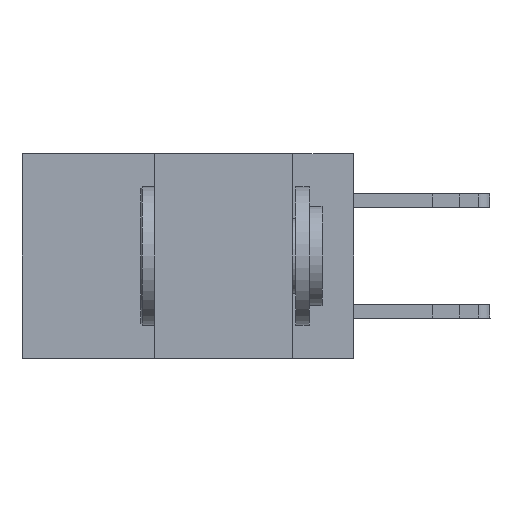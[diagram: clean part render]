
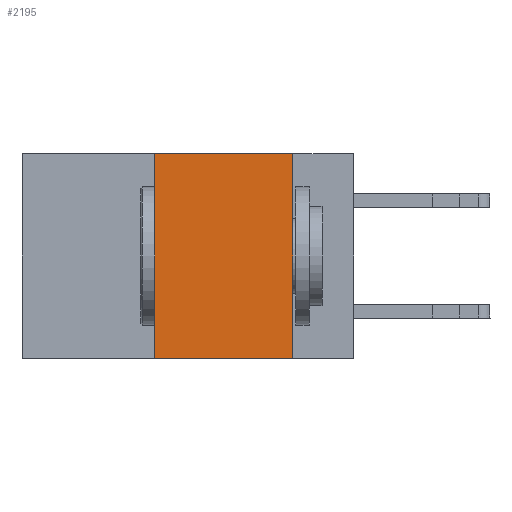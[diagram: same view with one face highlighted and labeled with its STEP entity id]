
A CAD part, left-side view. The second image highlights one B-rep face of the part: STEP entity #2195.
In plain terms, the highlighted planar face has unit normal (-1, 0, 0).
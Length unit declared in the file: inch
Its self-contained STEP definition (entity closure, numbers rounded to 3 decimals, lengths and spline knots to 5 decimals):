
#376 = DIRECTION ( 'NONE',  ( 0., 0., -1. ) ) ;
#899 = CARTESIAN_POINT ( 'NONE',  ( 0., 0.36, 0. ) ) ;
#1220 = VECTOR ( 'NONE', #376, 39.37008 ) ;
#1946 = LINE ( 'NONE', #11328, #1220 ) ;
#2195 = ADVANCED_FACE ( 'NONE', ( #16985 ), #2775, .F. ) ;
#2199 = VERTEX_POINT ( 'NONE', #9021 ) ;
#2643 = ORIENTED_EDGE ( 'NONE', *, *, #5644, .F. ) ;
#2775 = PLANE ( 'NONE',  #10626 ) ;
#2881 = CARTESIAN_POINT ( 'NONE',  ( 0., 0.36, -0.37 ) ) ;
#3214 = VERTEX_POINT ( 'NONE', #2881 ) ;
#4919 = VERTEX_POINT ( 'NONE', #899 ) ;
#5644 = EDGE_CURVE ( 'NONE', #3214, #4919, #19134, .T. ) ;
#6056 = CARTESIAN_POINT ( 'NONE',  ( 0., 0.36, 0. ) ) ;
#6963 = ORIENTED_EDGE ( 'NONE', *, *, #12796, .F. ) ;
#7498 = LINE ( 'NONE', #13873, #19566 ) ;
#8019 = EDGE_CURVE ( 'NONE', #3214, #10495, #7498, .T. ) ;
#8155 = EDGE_CURVE ( 'NONE', #2199, #10495, #1946, .T. ) ;
#8628 = LINE ( 'NONE', #11876, #16999 ) ;
#9021 = CARTESIAN_POINT ( 'NONE',  ( 0., 0.11, 0. ) ) ;
#10495 = VERTEX_POINT ( 'NONE', #16284 ) ;
#10577 = CARTESIAN_POINT ( 'NONE',  ( 0., 0.6, 0. ) ) ;
#10626 = AXIS2_PLACEMENT_3D ( 'NONE', #10577, #13936, #15633 ) ;
#11328 = CARTESIAN_POINT ( 'NONE',  ( 0., 0.11, 0. ) ) ;
#11876 = CARTESIAN_POINT ( 'NONE',  ( 0., 0.6, 0. ) ) ;
#12070 = EDGE_LOOP ( 'NONE', ( #12951, #6963, #2643, #18047 ) ) ;
#12796 = EDGE_CURVE ( 'NONE', #4919, #2199, #8628, .T. ) ;
#12951 = ORIENTED_EDGE ( 'NONE', *, *, #8155, .F. ) ;
#13873 = CARTESIAN_POINT ( 'NONE',  ( 0., 0.6, -0.37 ) ) ;
#13936 = DIRECTION ( 'NONE',  ( 1., 0., 0. ) ) ;
#15409 = VECTOR ( 'NONE', #18841, 39.37008 ) ;
#15633 = DIRECTION ( 'NONE',  ( 0., 0., -1. ) ) ;
#16284 = CARTESIAN_POINT ( 'NONE',  ( 0., 0.11, -0.37 ) ) ;
#16985 = FACE_OUTER_BOUND ( 'NONE', #12070, .T. ) ;
#16999 = VECTOR ( 'NONE', #19448, 39.37008 ) ;
#18047 = ORIENTED_EDGE ( 'NONE', *, *, #8019, .T. ) ;
#18720 = DIRECTION ( 'NONE',  ( 0., -1., 0. ) ) ;
#18841 = DIRECTION ( 'NONE',  ( 0., 0., 1. ) ) ;
#19134 = LINE ( 'NONE', #6056, #15409 ) ;
#19448 = DIRECTION ( 'NONE',  ( 0., -1., 0. ) ) ;
#19566 = VECTOR ( 'NONE', #18720, 39.37008 ) ;
